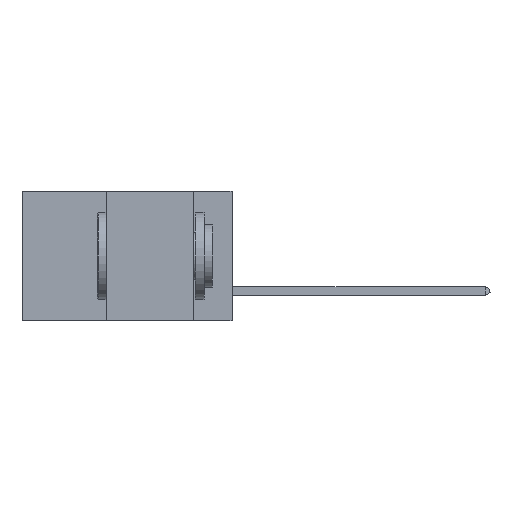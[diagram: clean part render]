
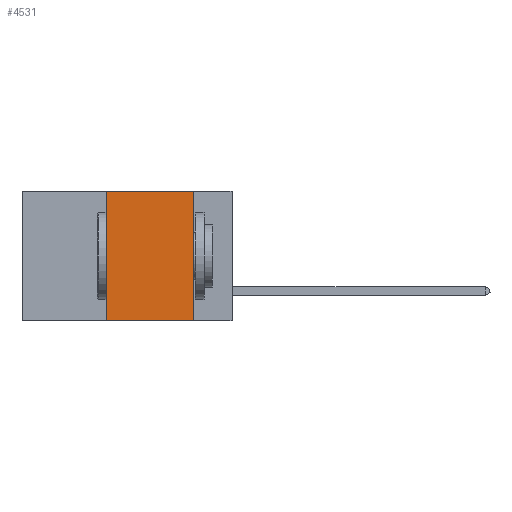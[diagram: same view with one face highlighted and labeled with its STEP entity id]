
A CAD part, left-side view. The second image highlights one B-rep face of the part: STEP entity #4531.
In plain terms, the highlighted planar face has unit normal (-1, 0, 0).
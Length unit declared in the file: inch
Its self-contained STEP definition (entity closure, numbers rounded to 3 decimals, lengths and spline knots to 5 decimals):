
#324 = EDGE_LOOP ( 'NONE', ( #2456, #11709, #12821, #21028 ) ) ;
#793 = VECTOR ( 'NONE', #14621, 39.37008 ) ;
#1258 = DIRECTION ( 'NONE',  ( 0., 0., -1. ) ) ;
#2056 = LINE ( 'NONE', #21408, #17527 ) ;
#2456 = ORIENTED_EDGE ( 'NONE', *, *, #18901, .F. ) ;
#2712 = FACE_OUTER_BOUND ( 'NONE', #324, .T. ) ;
#3415 = DIRECTION ( 'NONE',  ( 0., -1., 0. ) ) ;
#4193 = EDGE_CURVE ( 'NONE', #17871, #11449, #10500, .T. ) ;
#4280 = CARTESIAN_POINT ( 'NONE',  ( 0., 0.11, -0.37 ) ) ;
#4531 = ADVANCED_FACE ( 'NONE', ( #2712 ), #16775, .F. ) ;
#5769 = LINE ( 'NONE', #21189, #8101 ) ;
#6737 = CARTESIAN_POINT ( 'NONE',  ( 0., 0.6, 0. ) ) ;
#7490 = CARTESIAN_POINT ( 'NONE',  ( 0., 0.6, -0.37 ) ) ;
#8101 = VECTOR ( 'NONE', #1258, 39.37008 ) ;
#8328 = DIRECTION ( 'NONE',  ( 0., 0., -1. ) ) ;
#8399 = DIRECTION ( 'NONE',  ( 0., 0., 1. ) ) ;
#9177 = LINE ( 'NONE', #7490, #793 ) ;
#9220 = CARTESIAN_POINT ( 'NONE',  ( 0., 0.11, 0. ) ) ;
#9861 = VERTEX_POINT ( 'NONE', #20562 ) ;
#10500 = LINE ( 'NONE', #6737, #12921 ) ;
#11449 = VERTEX_POINT ( 'NONE', #9220 ) ;
#11565 = AXIS2_PLACEMENT_3D ( 'NONE', #11762, #20072, #8328 ) ;
#11709 = ORIENTED_EDGE ( 'NONE', *, *, #4193, .F. ) ;
#11762 = CARTESIAN_POINT ( 'NONE',  ( 0., 0.6, 0. ) ) ;
#12187 = CARTESIAN_POINT ( 'NONE',  ( 0., 0.36, 0. ) ) ;
#12821 = ORIENTED_EDGE ( 'NONE', *, *, #17639, .F. ) ;
#12921 = VECTOR ( 'NONE', #3415, 39.37008 ) ;
#14228 = VERTEX_POINT ( 'NONE', #4280 ) ;
#14621 = DIRECTION ( 'NONE',  ( 0., -1., 0. ) ) ;
#16671 = EDGE_CURVE ( 'NONE', #9861, #14228, #9177, .T. ) ;
#16775 = PLANE ( 'NONE',  #11565 ) ;
#17527 = VECTOR ( 'NONE', #8399, 39.37008 ) ;
#17639 = EDGE_CURVE ( 'NONE', #9861, #17871, #2056, .T. ) ;
#17871 = VERTEX_POINT ( 'NONE', #12187 ) ;
#18901 = EDGE_CURVE ( 'NONE', #11449, #14228, #5769, .T. ) ;
#20072 = DIRECTION ( 'NONE',  ( 1., 0., 0. ) ) ;
#20562 = CARTESIAN_POINT ( 'NONE',  ( 0., 0.36, -0.37 ) ) ;
#21028 = ORIENTED_EDGE ( 'NONE', *, *, #16671, .T. ) ;
#21189 = CARTESIAN_POINT ( 'NONE',  ( 0., 0.11, 0. ) ) ;
#21408 = CARTESIAN_POINT ( 'NONE',  ( 0., 0.36, 0. ) ) ;
